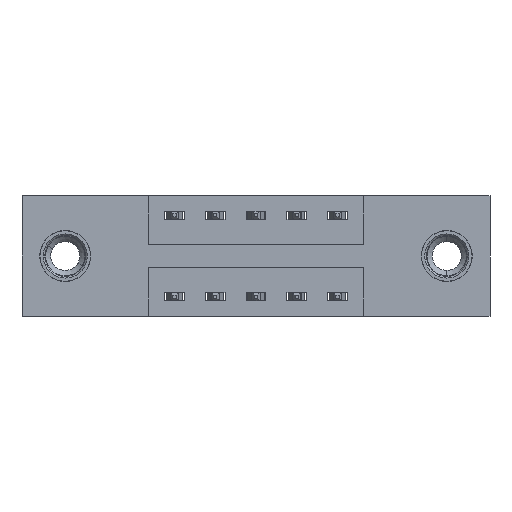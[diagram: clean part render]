
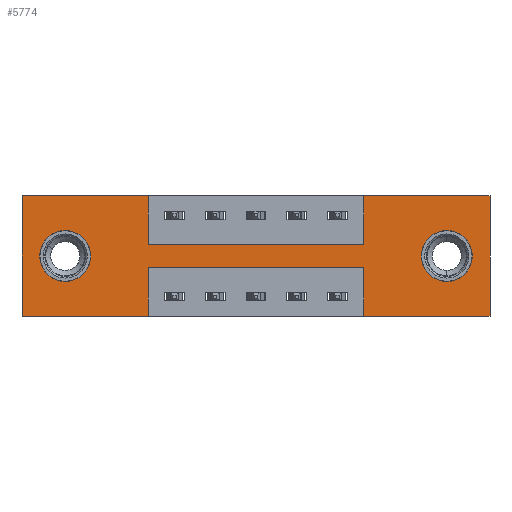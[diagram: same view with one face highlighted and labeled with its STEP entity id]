
A CAD part, front view. The second image highlights one B-rep face of the part: STEP entity #5774.
In plain terms, the highlighted planar face has unit normal (0, -1, 0).
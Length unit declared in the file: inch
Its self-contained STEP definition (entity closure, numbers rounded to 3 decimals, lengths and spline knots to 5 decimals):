
#64 = LINE ( 'NONE', #3149, #4187 ) ;
#76 = ORIENTED_EDGE ( 'NONE', *, *, #2049, .F. ) ;
#125 = LINE ( 'NONE', #6843, #1444 ) ;
#272 = CARTESIAN_POINT ( 'NONE',  ( 1.3025, 0., -0.185 ) ) ;
#294 = LINE ( 'NONE', #9050, #4495 ) ;
#363 = CARTESIAN_POINT ( 'NONE',  ( 0.3875, 0., 0. ) ) ;
#455 = VERTEX_POINT ( 'NONE', #1753 ) ;
#525 = CARTESIAN_POINT ( 'NONE',  ( 0., 0., 0. ) ) ;
#683 = EDGE_CURVE ( 'NONE', #4081, #7177, #4854, .T. ) ;
#692 = DIRECTION ( 'NONE',  ( -1., 0., 0. ) ) ;
#814 = EDGE_CURVE ( 'NONE', #905, #6117, #9470, .T. ) ;
#875 = CARTESIAN_POINT ( 'NONE',  ( 1.0475, 0., -0.22 ) ) ;
#905 = VERTEX_POINT ( 'NONE', #6942 ) ;
#911 = CARTESIAN_POINT ( 'NONE',  ( 0., 0., -0.37 ) ) ;
#1199 = EDGE_CURVE ( 'NONE', #6117, #905, #3228, .T. ) ;
#1268 = CARTESIAN_POINT ( 'NONE',  ( 0.3875, 0., -0.37 ) ) ;
#1429 = DIRECTION ( 'NONE',  ( 0., 0., 1. ) ) ;
#1444 = VECTOR ( 'NONE', #1681, 39.37008 ) ;
#1471 = ORIENTED_EDGE ( 'NONE', *, *, #7560, .F. ) ;
#1500 = DIRECTION ( 'NONE',  ( 0., 0., 1. ) ) ;
#1681 = DIRECTION ( 'NONE',  ( -1., 0., 0. ) ) ;
#1719 = PLANE ( 'NONE',  #3405 ) ;
#1753 = CARTESIAN_POINT ( 'NONE',  ( 0.3875, 0., 0. ) ) ;
#1817 = DIRECTION ( 'NONE',  ( 0., 0., -1. ) ) ;
#1927 = LINE ( 'NONE', #525, #4306 ) ;
#2021 = VERTEX_POINT ( 'NONE', #7604 ) ;
#2049 = EDGE_CURVE ( 'NONE', #6512, #8207, #1927, .T. ) ;
#2173 = CARTESIAN_POINT ( 'NONE',  ( 0.1325, 0., -0.185 ) ) ;
#2239 = CARTESIAN_POINT ( 'NONE',  ( 0.1325, 0., -0.185 ) ) ;
#2311 = FACE_BOUND ( 'NONE', #2997, .T. ) ;
#2384 = CARTESIAN_POINT ( 'NONE',  ( 1.435, 0., 0. ) ) ;
#2538 = ORIENTED_EDGE ( 'NONE', *, *, #5914, .F. ) ;
#2550 = DIRECTION ( 'NONE',  ( 1., 0., 0. ) ) ;
#2630 = EDGE_CURVE ( 'NONE', #2989, #5931, #9059, .T. ) ;
#2790 = DIRECTION ( 'NONE',  ( 1., 0., 0. ) ) ;
#2850 = ORIENTED_EDGE ( 'NONE', *, *, #6424, .F. ) ;
#2989 = VERTEX_POINT ( 'NONE', #8771 ) ;
#2997 = EDGE_LOOP ( 'NONE', ( #8112, #8640 ) ) ;
#3149 = CARTESIAN_POINT ( 'NONE',  ( 0.3875, 0., -0.15 ) ) ;
#3195 = ORIENTED_EDGE ( 'NONE', *, *, #683, .F. ) ;
#3228 = CIRCLE ( 'NONE', #9018, 0.078 ) ;
#3231 = DIRECTION ( 'NONE',  ( 0., 0., 1. ) ) ;
#3303 = LINE ( 'NONE', #363, #8625 ) ;
#3405 = AXIS2_PLACEMENT_3D ( 'NONE', #911, #5207, #3924 ) ;
#3411 = CARTESIAN_POINT ( 'NONE',  ( 1.0475, 0., 0. ) ) ;
#3474 = VECTOR ( 'NONE', #1429, 39.37008 ) ;
#3749 = DIRECTION ( 'NONE',  ( 0., 0., -1. ) ) ;
#3871 = DIRECTION ( 'NONE',  ( 0., 0., -1. ) ) ;
#3879 = CIRCLE ( 'NONE', #6776, 0.078 ) ;
#3924 = DIRECTION ( 'NONE',  ( 0., 0., -1. ) ) ;
#3943 = EDGE_CURVE ( 'NONE', #7009, #2021, #3879, .T. ) ;
#4006 = EDGE_CURVE ( 'NONE', #6314, #4290, #125, .T. ) ;
#4081 = VERTEX_POINT ( 'NONE', #875 ) ;
#4113 = CARTESIAN_POINT ( 'NONE',  ( 1.3025, 0., -0.107 ) ) ;
#4141 = CARTESIAN_POINT ( 'NONE',  ( 1.0475, 0., -0.15 ) ) ;
#4187 = VECTOR ( 'NONE', #8870, 39.37008 ) ;
#4290 = VERTEX_POINT ( 'NONE', #4975 ) ;
#4306 = VECTOR ( 'NONE', #2550, 39.37008 ) ;
#4339 = LINE ( 'NONE', #5150, #3474 ) ;
#4365 = DIRECTION ( 'NONE',  ( 0., 1., 0. ) ) ;
#4403 = CARTESIAN_POINT ( 'NONE',  ( 1.435, 0., 0. ) ) ;
#4418 = DIRECTION ( 'NONE',  ( 0., 1., 0. ) ) ;
#4449 = VERTEX_POINT ( 'NONE', #6862 ) ;
#4458 = EDGE_CURVE ( 'NONE', #5931, #4081, #294, .T. ) ;
#4495 = VECTOR ( 'NONE', #3231, 39.37008 ) ;
#4509 = VECTOR ( 'NONE', #5027, 39.37008 ) ;
#4516 = DIRECTION ( 'NONE',  ( 0., 0., 1. ) ) ;
#4550 = EDGE_LOOP ( 'NONE', ( #5237, #7415 ) ) ;
#4582 = ORIENTED_EDGE ( 'NONE', *, *, #4006, .F. ) ;
#4599 = VECTOR ( 'NONE', #692, 39.37008 ) ;
#4854 = LINE ( 'NONE', #5764, #4599 ) ;
#4880 = LINE ( 'NONE', #3411, #5882 ) ;
#4956 = ORIENTED_EDGE ( 'NONE', *, *, #7057, .F. ) ;
#4975 = CARTESIAN_POINT ( 'NONE',  ( 0., 0., -0.37 ) ) ;
#5027 = DIRECTION ( 'NONE',  ( 0., 0., -1. ) ) ;
#5150 = CARTESIAN_POINT ( 'NONE',  ( 0., 0., 0. ) ) ;
#5207 = DIRECTION ( 'NONE',  ( 0., -1., 0. ) ) ;
#5237 = ORIENTED_EDGE ( 'NONE', *, *, #814, .T. ) ;
#5437 = DIRECTION ( 'NONE',  ( -1., 0., 0. ) ) ;
#5490 = DIRECTION ( 'NONE',  ( 0., 0., -1. ) ) ;
#5599 = EDGE_CURVE ( 'NONE', #8207, #2989, #6509, .T. ) ;
#5764 = CARTESIAN_POINT ( 'NONE',  ( 0.3875, 0., -0.22 ) ) ;
#5774 = ADVANCED_FACE ( 'NONE', ( #2311, #8211, #8834 ), #1719, .T. ) ;
#5882 = VECTOR ( 'NONE', #8509, 39.37008 ) ;
#5914 = EDGE_CURVE ( 'NONE', #7177, #6314, #8350, .T. ) ;
#5931 = VERTEX_POINT ( 'NONE', #8537 ) ;
#6117 = VERTEX_POINT ( 'NONE', #7117 ) ;
#6152 = CARTESIAN_POINT ( 'NONE',  ( 0., 0., -0.37 ) ) ;
#6267 = CARTESIAN_POINT ( 'NONE',  ( 0., 0., 0. ) ) ;
#6314 = VERTEX_POINT ( 'NONE', #1268 ) ;
#6424 = EDGE_CURVE ( 'NONE', #6869, #6627, #64, .T. ) ;
#6509 = LINE ( 'NONE', #4403, #4509 ) ;
#6512 = VERTEX_POINT ( 'NONE', #6732 ) ;
#6521 = ORIENTED_EDGE ( 'NONE', *, *, #4458, .F. ) ;
#6581 = AXIS2_PLACEMENT_3D ( 'NONE', #2239, #4418, #4516 ) ;
#6627 = VERTEX_POINT ( 'NONE', #4141 ) ;
#6732 = CARTESIAN_POINT ( 'NONE',  ( 1.0475, 0., 0. ) ) ;
#6776 = AXIS2_PLACEMENT_3D ( 'NONE', #272, #8886, #3749 ) ;
#6839 = ORIENTED_EDGE ( 'NONE', *, *, #2630, .F. ) ;
#6843 = CARTESIAN_POINT ( 'NONE',  ( 0., 0., -0.37 ) ) ;
#6862 = CARTESIAN_POINT ( 'NONE',  ( 0., 0., 0. ) ) ;
#6869 = VERTEX_POINT ( 'NONE', #9032 ) ;
#6942 = CARTESIAN_POINT ( 'NONE',  ( 0.1325, 0., -0.107 ) ) ;
#6974 = AXIS2_PLACEMENT_3D ( 'NONE', #8295, #7459, #3871 ) ;
#7002 = EDGE_CURVE ( 'NONE', #4449, #455, #7178, .T. ) ;
#7009 = VERTEX_POINT ( 'NONE', #4113 ) ;
#7054 = VECTOR ( 'NONE', #5437, 39.37008 ) ;
#7057 = EDGE_CURVE ( 'NONE', #6627, #6512, #4880, .T. ) ;
#7117 = CARTESIAN_POINT ( 'NONE',  ( 0.1325, 0., -0.263 ) ) ;
#7177 = VERTEX_POINT ( 'NONE', #9421 ) ;
#7178 = LINE ( 'NONE', #6267, #8453 ) ;
#7367 = EDGE_LOOP ( 'NONE', ( #2538, #3195, #6521, #6839, #8905, #76, #4956, #2850, #1471, #9306, #8873, #4582 ) ) ;
#7415 = ORIENTED_EDGE ( 'NONE', *, *, #1199, .T. ) ;
#7459 = DIRECTION ( 'NONE',  ( 0., 1., 0. ) ) ;
#7551 = VECTOR ( 'NONE', #1817, 39.37008 ) ;
#7560 = EDGE_CURVE ( 'NONE', #455, #6869, #3303, .T. ) ;
#7604 = CARTESIAN_POINT ( 'NONE',  ( 1.3025, 0., -0.263 ) ) ;
#7890 = CIRCLE ( 'NONE', #6974, 0.078 ) ;
#8112 = ORIENTED_EDGE ( 'NONE', *, *, #3943, .T. ) ;
#8207 = VERTEX_POINT ( 'NONE', #2384 ) ;
#8211 = FACE_BOUND ( 'NONE', #4550, .T. ) ;
#8295 = CARTESIAN_POINT ( 'NONE',  ( 1.3025, 0., -0.185 ) ) ;
#8350 = LINE ( 'NONE', #8438, #7551 ) ;
#8438 = CARTESIAN_POINT ( 'NONE',  ( 0.3875, 0., -0.37 ) ) ;
#8453 = VECTOR ( 'NONE', #2790, 39.37008 ) ;
#8509 = DIRECTION ( 'NONE',  ( 0., 0., 1. ) ) ;
#8537 = CARTESIAN_POINT ( 'NONE',  ( 1.0475, 0., -0.37 ) ) ;
#8625 = VECTOR ( 'NONE', #5490, 39.37008 ) ;
#8640 = ORIENTED_EDGE ( 'NONE', *, *, #9065, .T. ) ;
#8771 = CARTESIAN_POINT ( 'NONE',  ( 1.435, 0., -0.37 ) ) ;
#8834 = FACE_OUTER_BOUND ( 'NONE', #7367, .T. ) ;
#8870 = DIRECTION ( 'NONE',  ( 1., 0., 0. ) ) ;
#8873 = ORIENTED_EDGE ( 'NONE', *, *, #9449, .F. ) ;
#8886 = DIRECTION ( 'NONE',  ( 0., 1., 0. ) ) ;
#8905 = ORIENTED_EDGE ( 'NONE', *, *, #5599, .F. ) ;
#9018 = AXIS2_PLACEMENT_3D ( 'NONE', #2173, #4365, #1500 ) ;
#9032 = CARTESIAN_POINT ( 'NONE',  ( 0.3875, 0., -0.15 ) ) ;
#9050 = CARTESIAN_POINT ( 'NONE',  ( 1.0475, 0., -0.37 ) ) ;
#9059 = LINE ( 'NONE', #6152, #7054 ) ;
#9065 = EDGE_CURVE ( 'NONE', #2021, #7009, #7890, .T. ) ;
#9306 = ORIENTED_EDGE ( 'NONE', *, *, #7002, .F. ) ;
#9421 = CARTESIAN_POINT ( 'NONE',  ( 0.3875, 0., -0.22 ) ) ;
#9449 = EDGE_CURVE ( 'NONE', #4290, #4449, #4339, .T. ) ;
#9470 = CIRCLE ( 'NONE', #6581, 0.078 ) ;
